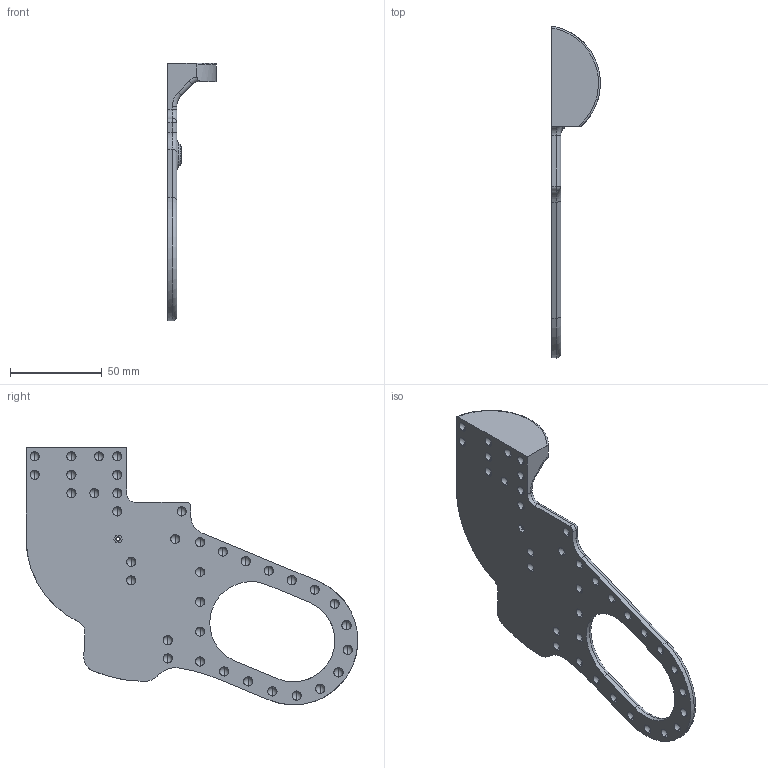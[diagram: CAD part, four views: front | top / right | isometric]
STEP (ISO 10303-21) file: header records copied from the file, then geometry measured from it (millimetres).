
FILE_DESCRIPTION (( 'STEP AP214' ), '1' );
FILE_NAME ('Side_Left.STEP', '2013-11-21T02:42:59', ( '' ), ( '' ), 'SwSTEP 2.0', 'SolidWorks 2013', '' );
FILE_SCHEMA (( 'AUTOMOTIVE_DESIGN' ));
Length unit declared in the file: millimetre
Products named in the file (1): Side_Left
Bounding box: 26.49 x 180.52 x 140.27 mm (x, y, z)
Volume: 71075.4 mm3; surface area: 30119.7 mm2
Topology: 1 solids, 1 shells, 152 faces, 448 edges, 264 vertices
Faces by surface type: sphere 73, cylinder 31, torus 25, plane 21, cone 2
Entity records: 4170 total; most frequent: DIRECTION 810, CARTESIAN_POINT 781, ORIENTED_EDGE 606, AXIS2_PLACEMENT_3D 366, EDGE_CURVE 303, CIRCLE 213, EDGE_LOOP 195, VERTEX_POINT 192
